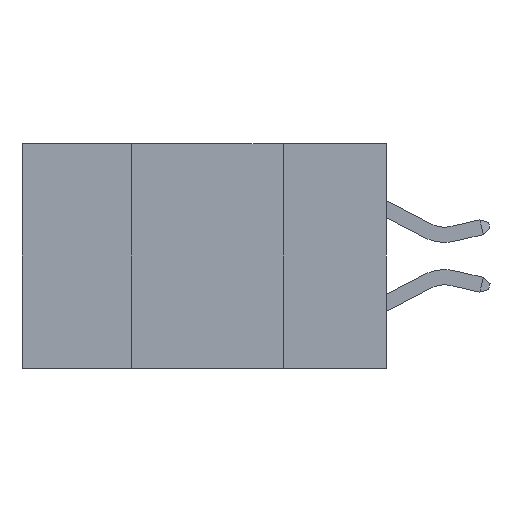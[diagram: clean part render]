
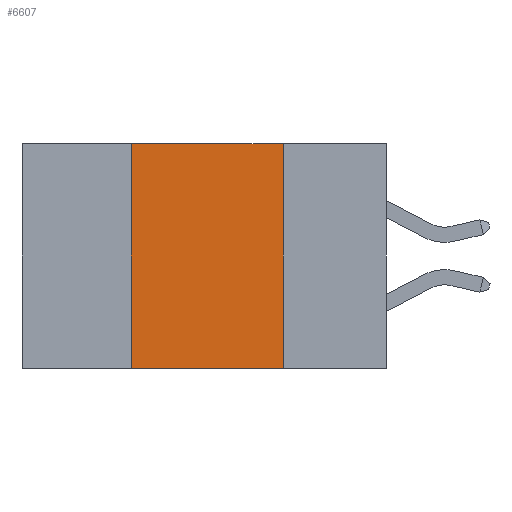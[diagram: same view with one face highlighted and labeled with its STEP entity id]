
A CAD part, left-side view. The second image highlights one B-rep face of the part: STEP entity #6607.
In plain terms, the highlighted planar face has unit normal (-1, 0, 0).
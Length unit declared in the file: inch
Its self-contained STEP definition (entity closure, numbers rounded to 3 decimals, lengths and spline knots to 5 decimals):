
#1064 = LINE ( 'NONE', #15331, #15454 ) ;
#1117 = LINE ( 'NONE', #14224, #15504 ) ;
#1340 = CARTESIAN_POINT ( 'NONE',  ( 0., 0.42, 0. ) ) ;
#1528 = DIRECTION ( 'NONE',  ( 0., 0., 1. ) ) ;
#3263 = ORIENTED_EDGE ( 'NONE', *, *, #15919, .F. ) ;
#3273 = LINE ( 'NONE', #14920, #18083 ) ;
#3473 = VECTOR ( 'NONE', #1528, 39.37008 ) ;
#5272 = EDGE_CURVE ( 'NONE', #16887, #13204, #1064, .T. ) ;
#5289 = AXIS2_PLACEMENT_3D ( 'NONE', #16266, #17576, #13475 ) ;
#5447 = CARTESIAN_POINT ( 'NONE',  ( 0., 0.17, -0.37 ) ) ;
#6069 = PLANE ( 'NONE',  #5289 ) ;
#6413 = DIRECTION ( 'NONE',  ( 0., -1., 0. ) ) ;
#6466 = ORIENTED_EDGE ( 'NONE', *, *, #5272, .F. ) ;
#6501 = CARTESIAN_POINT ( 'NONE',  ( 0., 0.42, 0. ) ) ;
#6607 = ADVANCED_FACE ( 'NONE', ( #16872 ), #6069, .F. ) ;
#8439 = DIRECTION ( 'NONE',  ( 0., 0., -1. ) ) ;
#8484 = CARTESIAN_POINT ( 'NONE',  ( 0., 0.17, 0. ) ) ;
#10166 = VERTEX_POINT ( 'NONE', #5447 ) ;
#11304 = ORIENTED_EDGE ( 'NONE', *, *, #12899, .T. ) ;
#12370 = EDGE_LOOP ( 'NONE', ( #3263, #6466, #17975, #11304 ) ) ;
#12899 = EDGE_CURVE ( 'NONE', #16541, #10166, #3273, .T. ) ;
#13204 = VERTEX_POINT ( 'NONE', #8484 ) ;
#13323 = EDGE_CURVE ( 'NONE', #16541, #16887, #17386, .T. ) ;
#13475 = DIRECTION ( 'NONE',  ( 0., 0., -1. ) ) ;
#14224 = CARTESIAN_POINT ( 'NONE',  ( 0., 0.17, 0. ) ) ;
#14920 = CARTESIAN_POINT ( 'NONE',  ( 0., 0.6, -0.37 ) ) ;
#15331 = CARTESIAN_POINT ( 'NONE',  ( 0., 0.6, 0. ) ) ;
#15454 = VECTOR ( 'NONE', #16645, 39.37008 ) ;
#15504 = VECTOR ( 'NONE', #8439, 39.37008 ) ;
#15583 = CARTESIAN_POINT ( 'NONE',  ( 0., 0.42, -0.37 ) ) ;
#15919 = EDGE_CURVE ( 'NONE', #13204, #10166, #1117, .T. ) ;
#16266 = CARTESIAN_POINT ( 'NONE',  ( 0., 0.6, 0. ) ) ;
#16541 = VERTEX_POINT ( 'NONE', #15583 ) ;
#16645 = DIRECTION ( 'NONE',  ( 0., -1., 0. ) ) ;
#16872 = FACE_OUTER_BOUND ( 'NONE', #12370, .T. ) ;
#16887 = VERTEX_POINT ( 'NONE', #6501 ) ;
#17386 = LINE ( 'NONE', #1340, #3473 ) ;
#17576 = DIRECTION ( 'NONE',  ( 1., 0., 0. ) ) ;
#17975 = ORIENTED_EDGE ( 'NONE', *, *, #13323, .F. ) ;
#18083 = VECTOR ( 'NONE', #6413, 39.37008 ) ;
